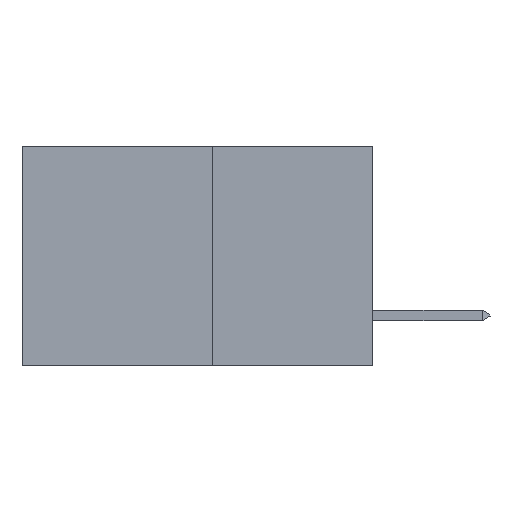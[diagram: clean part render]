
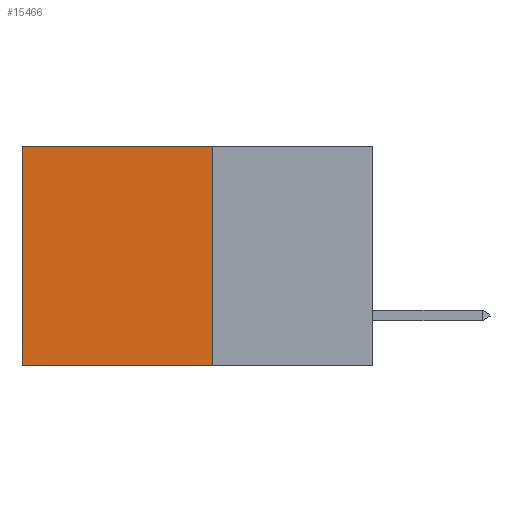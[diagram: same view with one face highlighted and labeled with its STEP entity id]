
A CAD part, left-side view. The second image highlights one B-rep face of the part: STEP entity #15466.
In plain terms, the highlighted planar face has unit normal (-1, 0, 0).
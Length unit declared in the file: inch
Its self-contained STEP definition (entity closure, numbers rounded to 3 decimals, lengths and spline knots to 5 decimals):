
#924 = ORIENTED_EDGE ( 'NONE', *, *, #6985, .F. ) ;
#1263 = DIRECTION ( 'NONE',  ( 0., 0., -1. ) ) ;
#2334 = CARTESIAN_POINT ( 'NONE',  ( 0.277, 0.27, -0.37 ) ) ;
#2357 = LINE ( 'NONE', #5485, #16072 ) ;
#2704 = CARTESIAN_POINT ( 'NONE',  ( 0.277, 0.27, -0.37 ) ) ;
#3822 = FACE_OUTER_BOUND ( 'NONE', #15907, .T. ) ;
#3836 = VECTOR ( 'NONE', #5367, 39.37008 ) ;
#4044 = CARTESIAN_POINT ( 'NONE',  ( 0.277, 0.27, 0. ) ) ;
#4062 = DIRECTION ( 'NONE',  ( 0., 1., 0. ) ) ;
#4247 = LINE ( 'NONE', #4044, #3836 ) ;
#4673 = CARTESIAN_POINT ( 'NONE',  ( 0.277, 0.59, -0.37 ) ) ;
#4785 = VERTEX_POINT ( 'NONE', #12337 ) ;
#4984 = EDGE_CURVE ( 'NONE', #5451, #15356, #15632, .T. ) ;
#5367 = DIRECTION ( 'NONE',  ( 0., 1., 0. ) ) ;
#5451 = VERTEX_POINT ( 'NONE', #11029 ) ;
#5485 = CARTESIAN_POINT ( 'NONE',  ( 0.277, 0.59, -0.37 ) ) ;
#5488 = ORIENTED_EDGE ( 'NONE', *, *, #4984, .F. ) ;
#6188 = DIRECTION ( 'NONE',  ( 0., 0., -1. ) ) ;
#6561 = PLANE ( 'NONE',  #13925 ) ;
#6822 = DIRECTION ( 'NONE',  ( 0., 0., -1. ) ) ;
#6985 = EDGE_CURVE ( 'NONE', #15356, #7275, #15772, .T. ) ;
#7275 = VERTEX_POINT ( 'NONE', #4673 ) ;
#9237 = DIRECTION ( 'NONE',  ( 1., 0., 0. ) ) ;
#9334 = ORIENTED_EDGE ( 'NONE', *, *, #13105, .T. ) ;
#11029 = CARTESIAN_POINT ( 'NONE',  ( 0.277, 0.27, 0. ) ) ;
#12337 = CARTESIAN_POINT ( 'NONE',  ( 0.277, 0.59, 0. ) ) ;
#12514 = VECTOR ( 'NONE', #6188, 39.37008 ) ;
#13105 = EDGE_CURVE ( 'NONE', #4785, #7275, #2357, .T. ) ;
#13925 = AXIS2_PLACEMENT_3D ( 'NONE', #17206, #9237, #1263 ) ;
#14136 = CARTESIAN_POINT ( 'NONE',  ( 0.277, 0.27, -0.37 ) ) ;
#14995 = EDGE_CURVE ( 'NONE', #5451, #4785, #4247, .T. ) ;
#15339 = VECTOR ( 'NONE', #4062, 39.37008 ) ;
#15356 = VERTEX_POINT ( 'NONE', #2334 ) ;
#15466 = ADVANCED_FACE ( 'NONE', ( #3822 ), #6561, .F. ) ;
#15632 = LINE ( 'NONE', #14136, #12514 ) ;
#15772 = LINE ( 'NONE', #2704, #15339 ) ;
#15907 = EDGE_LOOP ( 'NONE', ( #9334, #924, #5488, #17112 ) ) ;
#16072 = VECTOR ( 'NONE', #6822, 39.37008 ) ;
#17112 = ORIENTED_EDGE ( 'NONE', *, *, #14995, .T. ) ;
#17206 = CARTESIAN_POINT ( 'NONE',  ( 0.277, 0.27, -0.37 ) ) ;
